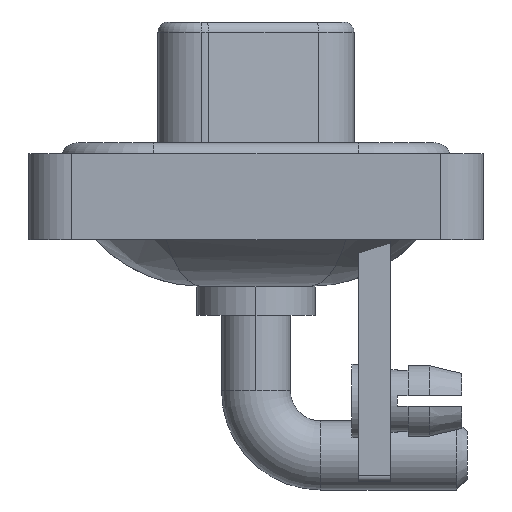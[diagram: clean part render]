
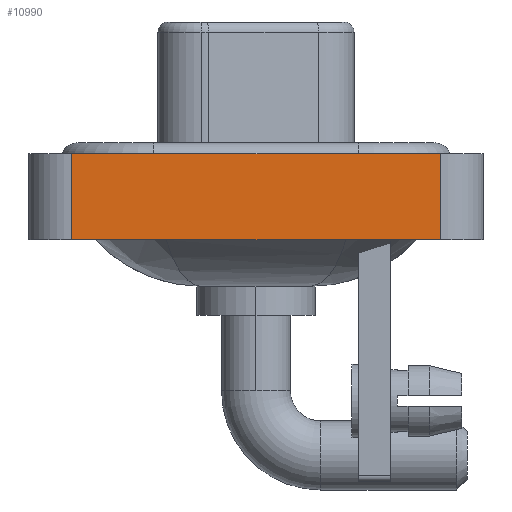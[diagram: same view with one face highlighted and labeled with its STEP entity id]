
A CAD part, left-side view. The second image highlights one B-rep face of the part: STEP entity #10990.
In plain terms, the highlighted planar face has unit normal (-1, 0, 0).
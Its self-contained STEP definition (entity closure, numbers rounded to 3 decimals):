
#306 = EDGE_CURVE ( 'NONE', #7736, #2401, #14840, .T. ) ;
#852 = LINE ( 'NONE', #10381, #2593 ) ;
#1174 = EDGE_LOOP ( 'NONE', ( #6376, #5663, #15767, #2489 ) ) ;
#2401 = VERTEX_POINT ( 'NONE', #10579 ) ;
#2473 = VECTOR ( 'NONE', #4095, 1000. ) ;
#2489 = ORIENTED_EDGE ( 'NONE', *, *, #4750, .T. ) ;
#2593 = VECTOR ( 'NONE', #9057, 1000. ) ;
#2738 = CARTESIAN_POINT ( 'NONE',  ( -7.25, 8.55, -3.6 ) ) ;
#3922 = CARTESIAN_POINT ( 'NONE',  ( -7.25, -8.55, -3.6 ) ) ;
#3932 = CARTESIAN_POINT ( 'NONE',  ( -7.25, -8.55, -3.6 ) ) ;
#4095 = DIRECTION ( 'NONE',  ( 0., -1., 0. ) ) ;
#4750 = EDGE_CURVE ( 'NONE', #7736, #11080, #7796, .T. ) ;
#4911 = FACE_OUTER_BOUND ( 'NONE', #1174, .T. ) ;
#5623 = LINE ( 'NONE', #13747, #16117 ) ;
#5663 = ORIENTED_EDGE ( 'NONE', *, *, #8186, .F. ) ;
#6144 = DIRECTION ( 'NONE',  ( -1., 0., 0. ) ) ;
#6376 = ORIENTED_EDGE ( 'NONE', *, *, #8080, .T. ) ;
#7466 = CARTESIAN_POINT ( 'NONE',  ( -7.25, -8.55, -3.6 ) ) ;
#7736 = VERTEX_POINT ( 'NONE', #14204 ) ;
#7796 = LINE ( 'NONE', #3922, #2473 ) ;
#8080 = EDGE_CURVE ( 'NONE', #11080, #10871, #5623, .T. ) ;
#8186 = EDGE_CURVE ( 'NONE', #2401, #10871, #852, .T. ) ;
#8725 = CARTESIAN_POINT ( 'NONE',  ( -7.25, -8.55, 0.4 ) ) ;
#9057 = DIRECTION ( 'NONE',  ( 0., -1., 0. ) ) ;
#9595 = DIRECTION ( 'NONE',  ( 0., 0., 1. ) ) ;
#9973 = AXIS2_PLACEMENT_3D ( 'NONE', #7466, #6144, #15688 ) ;
#10381 = CARTESIAN_POINT ( 'NONE',  ( -7.25, -8.55, 0.4 ) ) ;
#10579 = CARTESIAN_POINT ( 'NONE',  ( -7.25, 8.55, 0.4 ) ) ;
#10871 = VERTEX_POINT ( 'NONE', #8725 ) ;
#10990 = ADVANCED_FACE ( 'NONE', ( #4911 ), #17269, .T. ) ;
#11080 = VERTEX_POINT ( 'NONE', #3932 ) ;
#13747 = CARTESIAN_POINT ( 'NONE',  ( -7.25, -8.55, -3.6 ) ) ;
#14204 = CARTESIAN_POINT ( 'NONE',  ( -7.25, 8.55, -3.6 ) ) ;
#14350 = VECTOR ( 'NONE', #14751, 1000. ) ;
#14751 = DIRECTION ( 'NONE',  ( 0., 0., 1. ) ) ;
#14840 = LINE ( 'NONE', #2738, #14350 ) ;
#15688 = DIRECTION ( 'NONE',  ( 0., 0., 1. ) ) ;
#15767 = ORIENTED_EDGE ( 'NONE', *, *, #306, .F. ) ;
#16117 = VECTOR ( 'NONE', #9595, 1000. ) ;
#17269 = PLANE ( 'NONE',  #9973 ) ;
